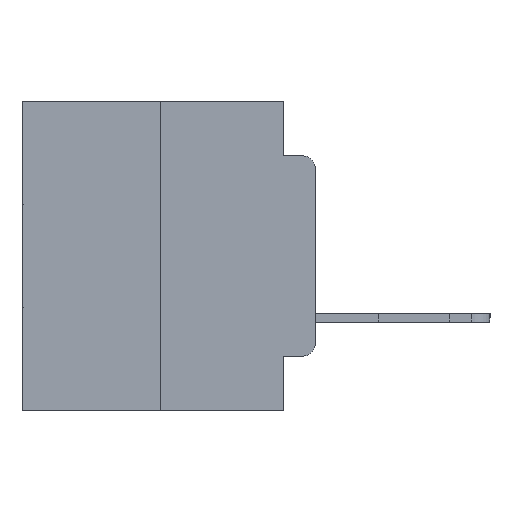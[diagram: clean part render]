
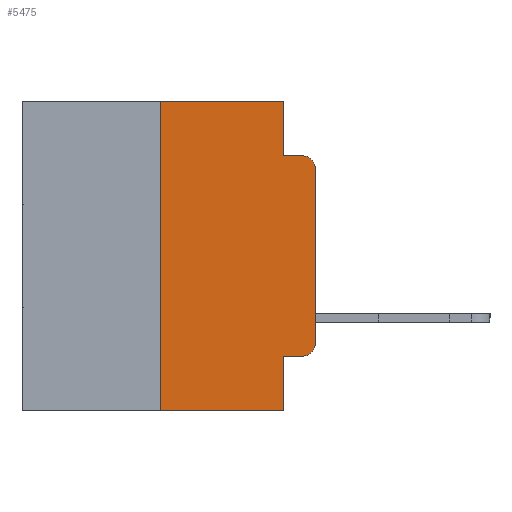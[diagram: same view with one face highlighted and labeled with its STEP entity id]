
A CAD part, left-side view. The second image highlights one B-rep face of the part: STEP entity #5475.
In plain terms, the highlighted planar face has unit normal (-1, 0, 0).
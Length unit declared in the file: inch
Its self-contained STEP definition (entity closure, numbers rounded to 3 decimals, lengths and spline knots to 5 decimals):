
#235 = DIRECTION ( 'NONE',  ( 0., 0., 1. ) ) ;
#405 = EDGE_CURVE ( 'NONE', #20179, #9883, #687, .T. ) ;
#509 = LINE ( 'NONE', #16668, #11818 ) ;
#687 = LINE ( 'NONE', #20956, #22568 ) ;
#1021 = VERTEX_POINT ( 'NONE', #27806 ) ;
#1080 = CARTESIAN_POINT ( 'NONE',  ( 0., 0.473, 0. ) ) ;
#1115 = CARTESIAN_POINT ( 'NONE',  ( 0., 0.02, -0.4115 ) ) ;
#1362 = ORIENTED_EDGE ( 'NONE', *, *, #2379, .F. ) ;
#1539 = CARTESIAN_POINT ( 'NONE',  ( 0., 0.25, 0. ) ) ;
#1971 = CARTESIAN_POINT ( 'NONE',  ( 0., 0., -0.1085 ) ) ;
#2268 = EDGE_CURVE ( 'NONE', #12593, #18687, #509, .T. ) ;
#2274 = EDGE_CURVE ( 'NONE', #18687, #27938, #6111, .T. ) ;
#2320 = EDGE_CURVE ( 'NONE', #17522, #27938, #5394, .T. ) ;
#2322 = EDGE_CURVE ( 'NONE', #1021, #17522, #20422, .T. ) ;
#2328 = AXIS2_PLACEMENT_3D ( 'NONE', #1080, #18672, #5884 ) ;
#2373 = EDGE_CURVE ( 'NONE', #20179, #11350, #14142, .T. ) ;
#2379 = EDGE_CURVE ( 'NONE', #26323, #9883, #24001, .T. ) ;
#2408 = EDGE_CURVE ( 'NONE', #26323, #15622, #12786, .T. ) ;
#2419 = EDGE_CURVE ( 'NONE', #15622, #12593, #22727, .T. ) ;
#3696 = VECTOR ( 'NONE', #9114, 39.37008 ) ;
#3832 = ORIENTED_EDGE ( 'NONE', *, *, #15989, .F. ) ;
#3885 = VECTOR ( 'NONE', #13505, 39.37008 ) ;
#3899 = ORIENTED_EDGE ( 'NONE', *, *, #2419, .T. ) ;
#4971 = CARTESIAN_POINT ( 'NONE',  ( 0., 0.051, -0.4115 ) ) ;
#5280 = DIRECTION ( 'NONE',  ( 0., 0., -1. ) ) ;
#5351 = DIRECTION ( 'NONE',  ( 0., -1., 0. ) ) ;
#5394 = LINE ( 'NONE', #14438, #3885 ) ;
#5475 = ADVANCED_FACE ( 'NONE', ( #15760 ), #14401, .F. ) ;
#5884 = DIRECTION ( 'NONE',  ( 0., 0., -1. ) ) ;
#5895 = DIRECTION ( 'NONE',  ( 0., 0., -1. ) ) ;
#6111 = CIRCLE ( 'NONE', #15305, 0.02 ) ;
#7028 = CARTESIAN_POINT ( 'NONE',  ( 0., 0.25, 0. ) ) ;
#7114 = CARTESIAN_POINT ( 'NONE',  ( 0., 0.051, 0. ) ) ;
#9114 = DIRECTION ( 'NONE',  ( 0., -1., 0. ) ) ;
#9883 = VERTEX_POINT ( 'NONE', #15019 ) ;
#10667 = ORIENTED_EDGE ( 'NONE', *, *, #2274, .T. ) ;
#10781 = ORIENTED_EDGE ( 'NONE', *, *, #405, .T. ) ;
#11350 = VERTEX_POINT ( 'NONE', #1539 ) ;
#11818 = VECTOR ( 'NONE', #16962, 39.37008 ) ;
#12593 = VERTEX_POINT ( 'NONE', #27421 ) ;
#12786 = LINE ( 'NONE', #4971, #17789 ) ;
#13030 = DIRECTION ( 'NONE',  ( -1., 0., 0. ) ) ;
#13099 = CARTESIAN_POINT ( 'NONE',  ( 0., 0.02, -0.3915 ) ) ;
#13451 = CARTESIAN_POINT ( 'NONE',  ( 0., 0.25, -0.5 ) ) ;
#13505 = DIRECTION ( 'NONE',  ( 0., -1., 0. ) ) ;
#14142 = LINE ( 'NONE', #7028, #19104 ) ;
#14401 = PLANE ( 'NONE',  #2328 ) ;
#14438 = CARTESIAN_POINT ( 'NONE',  ( 0., 0.051, -0.0885 ) ) ;
#14778 = VECTOR ( 'NONE', #5895, 39.37008 ) ;
#14874 = ORIENTED_EDGE ( 'NONE', *, *, #2320, .F. ) ;
#15019 = CARTESIAN_POINT ( 'NONE',  ( 0., 0.051, -0.5 ) ) ;
#15305 = AXIS2_PLACEMENT_3D ( 'NONE', #22307, #21868, #21846 ) ;
#15622 = VERTEX_POINT ( 'NONE', #1115 ) ;
#15760 = FACE_OUTER_BOUND ( 'NONE', #20002, .T. ) ;
#15989 = EDGE_CURVE ( 'NONE', #11350, #1021, #20245, .T. ) ;
#16668 = CARTESIAN_POINT ( 'NONE',  ( 0., 0., 0. ) ) ;
#16675 = ORIENTED_EDGE ( 'NONE', *, *, #2408, .T. ) ;
#16962 = DIRECTION ( 'NONE',  ( 0., 0., 1. ) ) ;
#17522 = VERTEX_POINT ( 'NONE', #26269 ) ;
#17591 = CARTESIAN_POINT ( 'NONE',  ( 0., 0.051, 0. ) ) ;
#17789 = VECTOR ( 'NONE', #5351, 39.37008 ) ;
#18462 = VECTOR ( 'NONE', #20828, 39.37008 ) ;
#18626 = CARTESIAN_POINT ( 'NONE',  ( 0., 0.051, -0.4115 ) ) ;
#18672 = DIRECTION ( 'NONE',  ( 1., 0., 0. ) ) ;
#18687 = VERTEX_POINT ( 'NONE', #1971 ) ;
#19104 = VECTOR ( 'NONE', #235, 39.37008 ) ;
#19877 = CARTESIAN_POINT ( 'NONE',  ( 0., 0.02, -0.0885 ) ) ;
#20002 = EDGE_LOOP ( 'NONE', ( #22263, #10667, #14874, #25074, #3832, #20729, #10781, #1362, #16675, #3899 ) ) ;
#20179 = VERTEX_POINT ( 'NONE', #13451 ) ;
#20245 = LINE ( 'NONE', #21801, #3696 ) ;
#20422 = LINE ( 'NONE', #17591, #14778 ) ;
#20729 = ORIENTED_EDGE ( 'NONE', *, *, #2373, .F. ) ;
#20828 = DIRECTION ( 'NONE',  ( 0., 0., -1. ) ) ;
#20956 = CARTESIAN_POINT ( 'NONE',  ( 0., 0.473, -0.5 ) ) ;
#21801 = CARTESIAN_POINT ( 'NONE',  ( 0., 0.473, 0. ) ) ;
#21846 = DIRECTION ( 'NONE',  ( 0., 0., -1. ) ) ;
#21868 = DIRECTION ( 'NONE',  ( -1., 0., 0. ) ) ;
#22263 = ORIENTED_EDGE ( 'NONE', *, *, #2268, .T. ) ;
#22307 = CARTESIAN_POINT ( 'NONE',  ( 0., 0.02, -0.1085 ) ) ;
#22568 = VECTOR ( 'NONE', #22801, 39.37008 ) ;
#22727 = CIRCLE ( 'NONE', #26593, 0.02 ) ;
#22801 = DIRECTION ( 'NONE',  ( 0., -1., 0. ) ) ;
#24001 = LINE ( 'NONE', #7114, #18462 ) ;
#25074 = ORIENTED_EDGE ( 'NONE', *, *, #2322, .F. ) ;
#26269 = CARTESIAN_POINT ( 'NONE',  ( 0., 0.051, -0.0885 ) ) ;
#26323 = VERTEX_POINT ( 'NONE', #18626 ) ;
#26593 = AXIS2_PLACEMENT_3D ( 'NONE', #13099, #13030, #5280 ) ;
#27421 = CARTESIAN_POINT ( 'NONE',  ( 0., 0., -0.3915 ) ) ;
#27806 = CARTESIAN_POINT ( 'NONE',  ( 0., 0.051, 0. ) ) ;
#27938 = VERTEX_POINT ( 'NONE', #19877 ) ;
